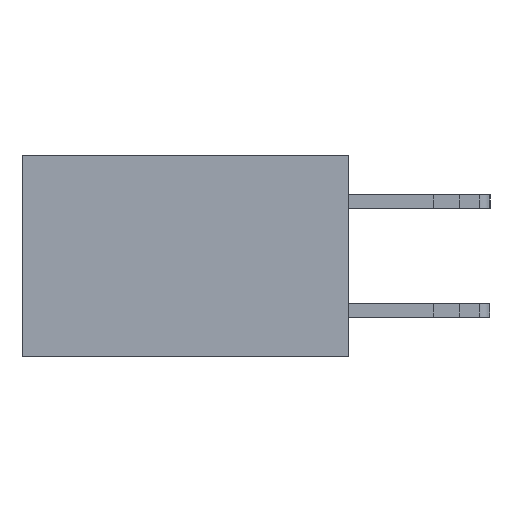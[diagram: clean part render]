
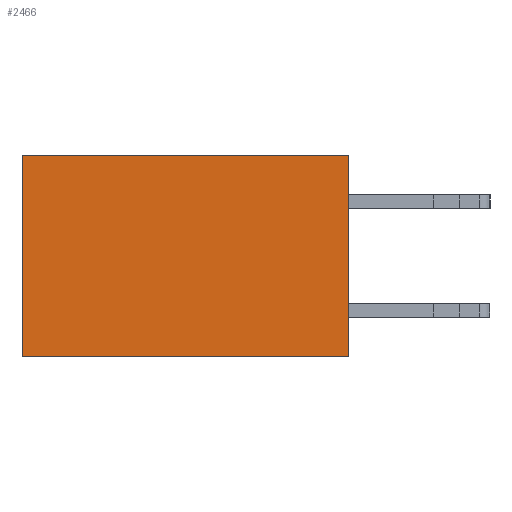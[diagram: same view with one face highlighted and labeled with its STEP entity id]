
A CAD part, left-side view. The second image highlights one B-rep face of the part: STEP entity #2466.
In plain terms, the highlighted planar face has unit normal (-1, 0, 0).
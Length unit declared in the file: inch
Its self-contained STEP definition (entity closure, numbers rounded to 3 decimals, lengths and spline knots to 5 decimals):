
#854 = EDGE_LOOP ( 'NONE', ( #11201, #7079, #21059, #20361 ) ) ;
#1854 = CARTESIAN_POINT ( 'NONE',  ( 0.298, 0.6, 0. ) ) ;
#2179 = VERTEX_POINT ( 'NONE', #1854 ) ;
#2241 = VECTOR ( 'NONE', #18451, 39.37008 ) ;
#2359 = VECTOR ( 'NONE', #11981, 39.37008 ) ;
#2466 = ADVANCED_FACE ( 'NONE', ( #10733 ), #10290, .F. ) ;
#2760 = CARTESIAN_POINT ( 'NONE',  ( 0.298, 0.6, 0. ) ) ;
#4673 = AXIS2_PLACEMENT_3D ( 'NONE', #23220, #11869, #11900 ) ;
#7079 = ORIENTED_EDGE ( 'NONE', *, *, #19253, .F. ) ;
#8310 = VERTEX_POINT ( 'NONE', #18690 ) ;
#8382 = LINE ( 'NONE', #12265, #2241 ) ;
#10222 = EDGE_CURVE ( 'NONE', #22459, #8310, #13356, .T. ) ;
#10290 = PLANE ( 'NONE',  #4673 ) ;
#10733 = FACE_OUTER_BOUND ( 'NONE', #854, .T. ) ;
#10875 = VECTOR ( 'NONE', #21276, 39.37008 ) ;
#11201 = ORIENTED_EDGE ( 'NONE', *, *, #21105, .T. ) ;
#11675 = DIRECTION ( 'NONE',  ( 0., 1., 0. ) ) ;
#11869 = DIRECTION ( 'NONE',  ( 1., 0., 0. ) ) ;
#11900 = DIRECTION ( 'NONE',  ( 0., 0., -1. ) ) ;
#11981 = DIRECTION ( 'NONE',  ( 0., 0., -1. ) ) ;
#12265 = CARTESIAN_POINT ( 'NONE',  ( 0.298, 0., -0.37 ) ) ;
#13356 = LINE ( 'NONE', #17982, #2359 ) ;
#15426 = VERTEX_POINT ( 'NONE', #19331 ) ;
#16352 = LINE ( 'NONE', #2760, #10875 ) ;
#17982 = CARTESIAN_POINT ( 'NONE',  ( 0.298, 0., 0. ) ) ;
#18451 = DIRECTION ( 'NONE',  ( 0., 1., 0. ) ) ;
#18690 = CARTESIAN_POINT ( 'NONE',  ( 0.298, 0., -0.37 ) ) ;
#19253 = EDGE_CURVE ( 'NONE', #8310, #15426, #8382, .T. ) ;
#19331 = CARTESIAN_POINT ( 'NONE',  ( 0.298, 0.6, -0.37 ) ) ;
#19932 = LINE ( 'NONE', #21875, #21203 ) ;
#20313 = EDGE_CURVE ( 'NONE', #22459, #2179, #19932, .T. ) ;
#20361 = ORIENTED_EDGE ( 'NONE', *, *, #20313, .T. ) ;
#21059 = ORIENTED_EDGE ( 'NONE', *, *, #10222, .F. ) ;
#21105 = EDGE_CURVE ( 'NONE', #2179, #15426, #16352, .T. ) ;
#21124 = CARTESIAN_POINT ( 'NONE',  ( 0.298, 0., 0. ) ) ;
#21203 = VECTOR ( 'NONE', #11675, 39.37008 ) ;
#21276 = DIRECTION ( 'NONE',  ( 0., 0., -1. ) ) ;
#21875 = CARTESIAN_POINT ( 'NONE',  ( 0.298, 0., 0. ) ) ;
#22459 = VERTEX_POINT ( 'NONE', #21124 ) ;
#23220 = CARTESIAN_POINT ( 'NONE',  ( 0.298, 0., 0. ) ) ;
